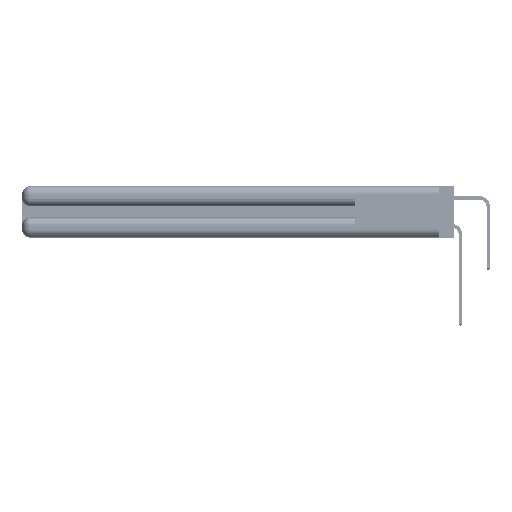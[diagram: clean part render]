
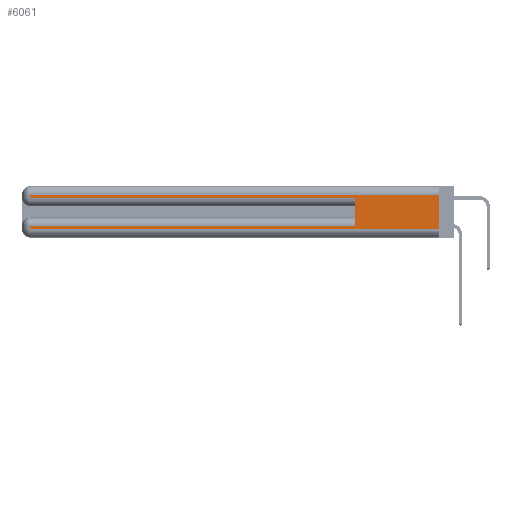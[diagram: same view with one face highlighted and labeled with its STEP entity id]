
A CAD part, left-side view. The second image highlights one B-rep face of the part: STEP entity #6061.
In plain terms, the highlighted planar face has unit normal (-1, 0, 0).
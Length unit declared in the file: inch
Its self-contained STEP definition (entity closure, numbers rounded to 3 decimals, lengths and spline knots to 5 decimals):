
#36 = ORIENTED_EDGE ( 'NONE', *, *, #25006, .T. ) ;
#179 = EDGE_CURVE ( 'NONE', #49272, #28694, #47914, .T. ) ;
#1117 = VECTOR ( 'NONE', #36200, 39.37008 ) ;
#1252 = EDGE_CURVE ( 'NONE', #37328, #49999, #10513, .T. ) ;
#3070 = CARTESIAN_POINT ( 'NONE',  ( 0., 0.6, 0.145 ) ) ;
#3314 = DIRECTION ( 'NONE',  ( 0., 0., -1. ) ) ;
#3436 = VERTEX_POINT ( 'NONE', #18691 ) ;
#3830 = VECTOR ( 'NONE', #44897, 39.37008 ) ;
#4093 = DIRECTION ( 'NONE',  ( 1., 0., 0. ) ) ;
#4193 = LINE ( 'NONE', #24372, #46156 ) ;
#4786 = VECTOR ( 'NONE', #38035, 39.37008 ) ;
#6059 = ORIENTED_EDGE ( 'NONE', *, *, #1252, .T. ) ;
#6061 = ADVANCED_FACE ( 'NONE', ( #25658 ), #54190, .F. ) ;
#6138 = LINE ( 'NONE', #42192, #4786 ) ;
#6364 = CARTESIAN_POINT ( 'NONE',  ( 0., 2.94, 0.06 ) ) ;
#6960 = EDGE_CURVE ( 'NONE', #37328, #3436, #24986, .T. ) ;
#9033 = CARTESIAN_POINT ( 'NONE',  ( 0., 0., 0.285 ) ) ;
#10513 = LINE ( 'NONE', #29044, #31540 ) ;
#11304 = VERTEX_POINT ( 'NONE', #14164 ) ;
#12478 = CARTESIAN_POINT ( 'NONE',  ( 0., 0., 0.37 ) ) ;
#12814 = CARTESIAN_POINT ( 'NONE',  ( 0., 0.6, 0.085 ) ) ;
#14164 = CARTESIAN_POINT ( 'NONE',  ( 0., 2.94, 0.31 ) ) ;
#16220 = VECTOR ( 'NONE', #29986, 39.37008 ) ;
#18353 = CARTESIAN_POINT ( 'NONE',  ( 0., 2.94, 0.285 ) ) ;
#18533 = CARTESIAN_POINT ( 'NONE',  ( 0., 0., 0.37 ) ) ;
#18691 = CARTESIAN_POINT ( 'NONE',  ( 0., 0.6, 0.285 ) ) ;
#21190 = ORIENTED_EDGE ( 'NONE', *, *, #51842, .T. ) ;
#22173 = EDGE_CURVE ( 'NONE', #30137, #28694, #23631, .T. ) ;
#22778 = CARTESIAN_POINT ( 'NONE',  ( 0., 2.94, 0.085 ) ) ;
#23439 = LINE ( 'NONE', #25901, #44322 ) ;
#23631 = LINE ( 'NONE', #32012, #1117 ) ;
#23932 = EDGE_CURVE ( 'NONE', #53689, #3436, #38474, .T. ) ;
#24372 = CARTESIAN_POINT ( 'NONE',  ( 0., 2.94, 0.37 ) ) ;
#24986 = LINE ( 'NONE', #3070, #3830 ) ;
#25006 = EDGE_CURVE ( 'NONE', #49999, #30137, #4193, .T. ) ;
#25034 = DIRECTION ( 'NONE',  ( 0., 1., 0. ) ) ;
#25658 = FACE_OUTER_BOUND ( 'NONE', #50929, .T. ) ;
#25901 = CARTESIAN_POINT ( 'NONE',  ( 0., 0., 0.31 ) ) ;
#25961 = CARTESIAN_POINT ( 'NONE',  ( 0., 0., 0.31 ) ) ;
#28694 = VERTEX_POINT ( 'NONE', #46901 ) ;
#29044 = CARTESIAN_POINT ( 'NONE',  ( 0., 0., 0.085 ) ) ;
#29986 = DIRECTION ( 'NONE',  ( 0., -1., 0. ) ) ;
#30110 = DIRECTION ( 'NONE',  ( 0., 1., 0. ) ) ;
#30137 = VERTEX_POINT ( 'NONE', #6364 ) ;
#31167 = DIRECTION ( 'NONE',  ( 0., 0., -1. ) ) ;
#31540 = VECTOR ( 'NONE', #25034, 39.37008 ) ;
#32012 = CARTESIAN_POINT ( 'NONE',  ( 0., 0., 0.06 ) ) ;
#32350 = ORIENTED_EDGE ( 'NONE', *, *, #32360, .T. ) ;
#32360 = EDGE_CURVE ( 'NONE', #11304, #53689, #6138, .T. ) ;
#33572 = DIRECTION ( 'NONE',  ( 0., 0., -1. ) ) ;
#36200 = DIRECTION ( 'NONE',  ( 0., -1., 0. ) ) ;
#36846 = VECTOR ( 'NONE', #31167, 39.37008 ) ;
#37328 = VERTEX_POINT ( 'NONE', #12814 ) ;
#37624 = ORIENTED_EDGE ( 'NONE', *, *, #22173, .T. ) ;
#38035 = DIRECTION ( 'NONE',  ( 0., 0., -1. ) ) ;
#38474 = LINE ( 'NONE', #9033, #16220 ) ;
#39524 = ORIENTED_EDGE ( 'NONE', *, *, #179, .F. ) ;
#42192 = CARTESIAN_POINT ( 'NONE',  ( 0., 2.94, 0.37 ) ) ;
#44322 = VECTOR ( 'NONE', #30110, 39.37008 ) ;
#44897 = DIRECTION ( 'NONE',  ( 0., 0., 1. ) ) ;
#45283 = AXIS2_PLACEMENT_3D ( 'NONE', #12478, #4093, #33572 ) ;
#46156 = VECTOR ( 'NONE', #3314, 39.37008 ) ;
#46901 = CARTESIAN_POINT ( 'NONE',  ( 0., 0., 0.06 ) ) ;
#47310 = ORIENTED_EDGE ( 'NONE', *, *, #23932, .T. ) ;
#47914 = LINE ( 'NONE', #18533, #36846 ) ;
#49266 = ORIENTED_EDGE ( 'NONE', *, *, #6960, .F. ) ;
#49272 = VERTEX_POINT ( 'NONE', #25961 ) ;
#49999 = VERTEX_POINT ( 'NONE', #22778 ) ;
#50929 = EDGE_LOOP ( 'NONE', ( #39524, #21190, #32350, #47310, #49266, #6059, #36, #37624 ) ) ;
#51842 = EDGE_CURVE ( 'NONE', #49272, #11304, #23439, .T. ) ;
#53689 = VERTEX_POINT ( 'NONE', #18353 ) ;
#54190 = PLANE ( 'NONE',  #45283 ) ;
